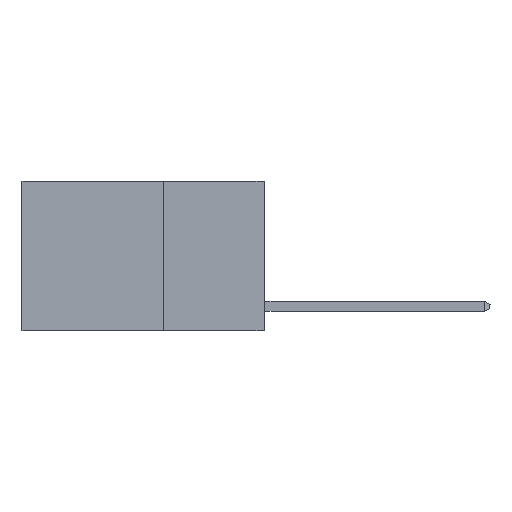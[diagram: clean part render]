
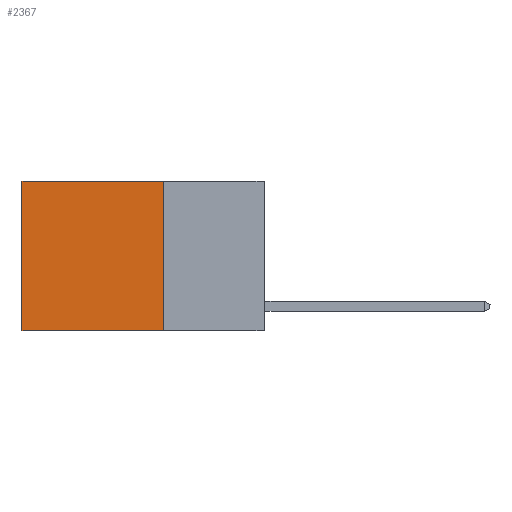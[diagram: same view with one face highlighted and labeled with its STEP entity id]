
A CAD part, left-side view. The second image highlights one B-rep face of the part: STEP entity #2367.
In plain terms, the highlighted planar face has unit normal (-1, 0, 0).
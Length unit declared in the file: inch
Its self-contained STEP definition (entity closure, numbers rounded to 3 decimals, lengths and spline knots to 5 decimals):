
#618 = LINE ( 'NONE', #11582, #2564 ) ;
#729 = EDGE_CURVE ( 'NONE', #12675, #22478, #9851, .T. ) ;
#1585 = CARTESIAN_POINT ( 'NONE',  ( 0.2625, 0.25, 0. ) ) ;
#2367 = ADVANCED_FACE ( 'NONE', ( #14555 ), #16561, .F. ) ;
#2564 = VECTOR ( 'NONE', #15258, 39.37008 ) ;
#2698 = LINE ( 'NONE', #17367, #2911 ) ;
#2791 = LINE ( 'NONE', #11987, #4229 ) ;
#2911 = VECTOR ( 'NONE', #13535, 39.37008 ) ;
#4229 = VECTOR ( 'NONE', #13882, 39.37008 ) ;
#4280 = ORIENTED_EDGE ( 'NONE', *, *, #14496, .T. ) ;
#4652 = VECTOR ( 'NONE', #19338, 39.37008 ) ;
#5119 = EDGE_CURVE ( 'NONE', #14816, #18067, #2791, .T. ) ;
#6635 = ORIENTED_EDGE ( 'NONE', *, *, #17250, .F. ) ;
#6816 = ORIENTED_EDGE ( 'NONE', *, *, #729, .F. ) ;
#9725 = CARTESIAN_POINT ( 'NONE',  ( 0.2625, 0.25, -0.37 ) ) ;
#9851 = LINE ( 'NONE', #22934, #4652 ) ;
#9945 = AXIS2_PLACEMENT_3D ( 'NONE', #1585, #12771, #18412 ) ;
#11582 = CARTESIAN_POINT ( 'NONE',  ( 0.2625, 0.25, -0.37 ) ) ;
#11987 = CARTESIAN_POINT ( 'NONE',  ( 0.2625, 0.6, 0. ) ) ;
#12675 = VERTEX_POINT ( 'NONE', #21442 ) ;
#12771 = DIRECTION ( 'NONE',  ( 1., 0., 0. ) ) ;
#13535 = DIRECTION ( 'NONE',  ( 0., 1., 0. ) ) ;
#13543 = ORIENTED_EDGE ( 'NONE', *, *, #5119, .T. ) ;
#13882 = DIRECTION ( 'NONE',  ( 0., 0., -1. ) ) ;
#14496 = EDGE_CURVE ( 'NONE', #12675, #14816, #2698, .T. ) ;
#14555 = FACE_OUTER_BOUND ( 'NONE', #22626, .T. ) ;
#14816 = VERTEX_POINT ( 'NONE', #17091 ) ;
#15258 = DIRECTION ( 'NONE',  ( 0., 1., 0. ) ) ;
#16561 = PLANE ( 'NONE',  #9945 ) ;
#17091 = CARTESIAN_POINT ( 'NONE',  ( 0.2625, 0.6, 0. ) ) ;
#17250 = EDGE_CURVE ( 'NONE', #22478, #18067, #618, .T. ) ;
#17367 = CARTESIAN_POINT ( 'NONE',  ( 0.2625, 0.25, 0. ) ) ;
#18067 = VERTEX_POINT ( 'NONE', #21187 ) ;
#18412 = DIRECTION ( 'NONE',  ( 0., 0., -1. ) ) ;
#19338 = DIRECTION ( 'NONE',  ( 0., 0., -1. ) ) ;
#21187 = CARTESIAN_POINT ( 'NONE',  ( 0.2625, 0.6, -0.37 ) ) ;
#21442 = CARTESIAN_POINT ( 'NONE',  ( 0.2625, 0.25, 0. ) ) ;
#22478 = VERTEX_POINT ( 'NONE', #9725 ) ;
#22626 = EDGE_LOOP ( 'NONE', ( #13543, #6635, #6816, #4280 ) ) ;
#22934 = CARTESIAN_POINT ( 'NONE',  ( 0.2625, 0.25, 0. ) ) ;
